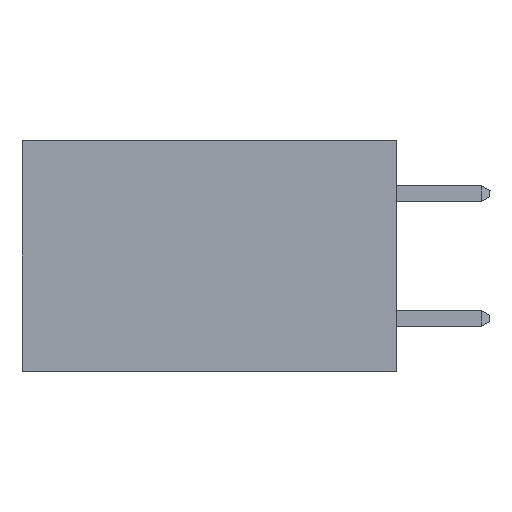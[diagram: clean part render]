
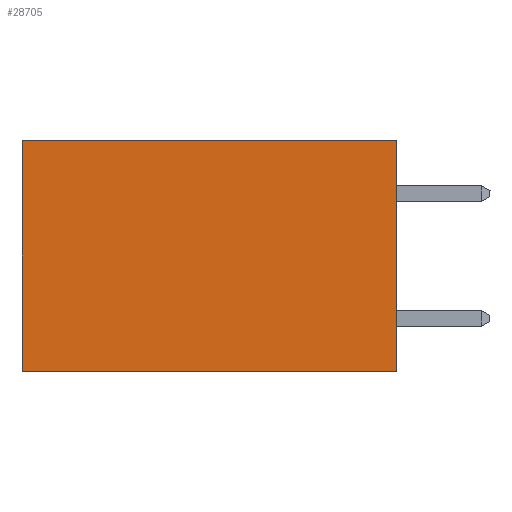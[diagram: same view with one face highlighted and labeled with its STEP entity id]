
A CAD part, left-side view. The second image highlights one B-rep face of the part: STEP entity #28705.
In plain terms, the highlighted planar face has unit normal (-1, 0, 0).
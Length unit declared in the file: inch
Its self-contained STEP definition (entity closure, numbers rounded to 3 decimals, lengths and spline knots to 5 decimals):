
#3362 = EDGE_LOOP ( 'NONE', ( #31115, #13135, #9804, #16115 ) ) ;
#5460 = LINE ( 'NONE', #27350, #30822 ) ;
#7610 = PLANE ( 'NONE',  #31335 ) ;
#7868 = EDGE_CURVE ( 'NONE', #27288, #16617, #5460, .T. ) ;
#8531 = CARTESIAN_POINT ( 'NONE',  ( 0.298, 0., 0. ) ) ;
#9804 = ORIENTED_EDGE ( 'NONE', *, *, #7868, .F. ) ;
#9979 = VECTOR ( 'NONE', #28425, 39.37008 ) ;
#9996 = CARTESIAN_POINT ( 'NONE',  ( 0.298, 0.6, -0.37 ) ) ;
#10190 = DIRECTION ( 'NONE',  ( 0., 0., -1. ) ) ;
#12614 = CARTESIAN_POINT ( 'NONE',  ( 0.298, 0., 0. ) ) ;
#12934 = LINE ( 'NONE', #16303, #18695 ) ;
#13135 = ORIENTED_EDGE ( 'NONE', *, *, #20723, .F. ) ;
#14046 = CARTESIAN_POINT ( 'NONE',  ( 0.298, 0., -0.37 ) ) ;
#15606 = VERTEX_POINT ( 'NONE', #9996 ) ;
#16115 = ORIENTED_EDGE ( 'NONE', *, *, #18064, .T. ) ;
#16256 = VECTOR ( 'NONE', #24485, 39.37008 ) ;
#16303 = CARTESIAN_POINT ( 'NONE',  ( 0.298, 0., 0. ) ) ;
#16617 = VERTEX_POINT ( 'NONE', #14046 ) ;
#17764 = CARTESIAN_POINT ( 'NONE',  ( 0.298, 0.6, 0. ) ) ;
#18064 = EDGE_CURVE ( 'NONE', #27288, #29389, #12934, .T. ) ;
#18695 = VECTOR ( 'NONE', #21045, 39.37008 ) ;
#20723 = EDGE_CURVE ( 'NONE', #16617, #15606, #29491, .T. ) ;
#20990 = EDGE_CURVE ( 'NONE', #29389, #15606, #29879, .T. ) ;
#21045 = DIRECTION ( 'NONE',  ( 0., 1., 0. ) ) ;
#24485 = DIRECTION ( 'NONE',  ( 0., 0., -1. ) ) ;
#24875 = DIRECTION ( 'NONE',  ( 1., 0., 0. ) ) ;
#25992 = CARTESIAN_POINT ( 'NONE',  ( 0.298, 0., -0.37 ) ) ;
#27288 = VERTEX_POINT ( 'NONE', #8531 ) ;
#27350 = CARTESIAN_POINT ( 'NONE',  ( 0.298, 0., 0. ) ) ;
#27391 = DIRECTION ( 'NONE',  ( 0., 0., -1. ) ) ;
#28425 = DIRECTION ( 'NONE',  ( 0., 1., 0. ) ) ;
#28705 = ADVANCED_FACE ( 'NONE', ( #30330 ), #7610, .F. ) ;
#29354 = CARTESIAN_POINT ( 'NONE',  ( 0.298, 0.6, 0. ) ) ;
#29389 = VERTEX_POINT ( 'NONE', #17764 ) ;
#29491 = LINE ( 'NONE', #25992, #9979 ) ;
#29879 = LINE ( 'NONE', #29354, #16256 ) ;
#30330 = FACE_OUTER_BOUND ( 'NONE', #3362, .T. ) ;
#30822 = VECTOR ( 'NONE', #27391, 39.37008 ) ;
#31115 = ORIENTED_EDGE ( 'NONE', *, *, #20990, .T. ) ;
#31335 = AXIS2_PLACEMENT_3D ( 'NONE', #12614, #24875, #10190 ) ;
